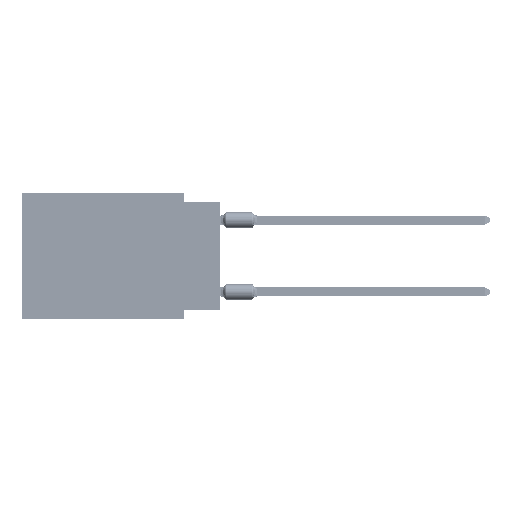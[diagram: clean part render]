
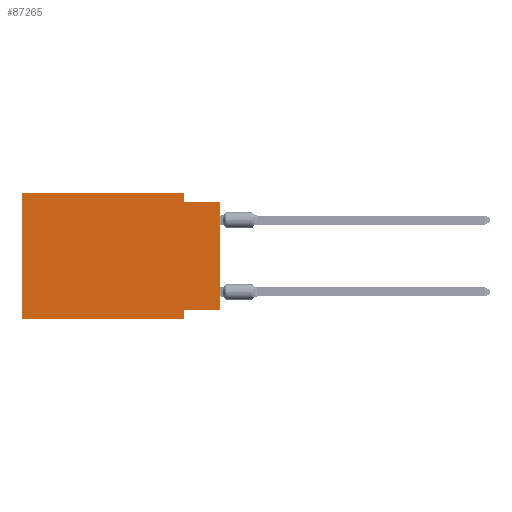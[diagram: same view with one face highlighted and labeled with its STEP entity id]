
A CAD part, left-side view. The second image highlights one B-rep face of the part: STEP entity #87265.
In plain terms, the highlighted planar face has unit normal (-1, 0, 0).
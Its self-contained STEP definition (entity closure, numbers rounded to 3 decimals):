
#952 = ORIENTED_EDGE ( 'NONE', *, *, #56576, .F. ) ;
#2219 = CARTESIAN_POINT ( 'NONE',  ( 0., 2.54, 0. ) ) ;
#2285 = LINE ( 'NONE', #32668, #85228 ) ;
#3794 = DIRECTION ( 'NONE',  ( 0., 0., -1. ) ) ;
#4928 = CARTESIAN_POINT ( 'NONE',  ( 0., 13.97, 0. ) ) ;
#5363 = VECTOR ( 'NONE', #19397, 1000. ) ;
#5784 = LINE ( 'NONE', #38015, #12832 ) ;
#7619 = EDGE_CURVE ( 'NONE', #47297, #87229, #2285, .T. ) ;
#8811 = VERTEX_POINT ( 'NONE', #83536 ) ;
#10686 = VECTOR ( 'NONE', #46884, 1000. ) ;
#11217 = DIRECTION ( 'NONE',  ( 0., 0., 1. ) ) ;
#11540 = VERTEX_POINT ( 'NONE', #43301 ) ;
#11664 = ORIENTED_EDGE ( 'NONE', *, *, #51901, .F. ) ;
#11834 = CARTESIAN_POINT ( 'NONE',  ( 0., 0., -8.255 ) ) ;
#12472 = ORIENTED_EDGE ( 'NONE', *, *, #55573, .F. ) ;
#12832 = VECTOR ( 'NONE', #90845, 1000. ) ;
#14168 = CARTESIAN_POINT ( 'NONE',  ( 0., 13.97, 0. ) ) ;
#14351 = LINE ( 'NONE', #88632, #70474 ) ;
#17151 = LINE ( 'NONE', #54526, #26824 ) ;
#19187 = CARTESIAN_POINT ( 'NONE',  ( 0., 13.97, -8.89 ) ) ;
#19397 = DIRECTION ( 'NONE',  ( 0., -1., 0. ) ) ;
#20477 = DIRECTION ( 'NONE',  ( 0., 0., -1. ) ) ;
#20645 = EDGE_CURVE ( 'NONE', #57954, #40935, #31451, .T. ) ;
#26824 = VECTOR ( 'NONE', #85425, 1000. ) ;
#27774 = EDGE_CURVE ( 'NONE', #8811, #11540, #42117, .T. ) ;
#30116 = EDGE_CURVE ( 'NONE', #36632, #11540, #65821, .T. ) ;
#31357 = ORIENTED_EDGE ( 'NONE', *, *, #20645, .F. ) ;
#31451 = LINE ( 'NONE', #38935, #10686 ) ;
#32668 = CARTESIAN_POINT ( 'NONE',  ( 0., 0., 0. ) ) ;
#36148 = DIRECTION ( 'NONE',  ( 1., 0., 0. ) ) ;
#36632 = VERTEX_POINT ( 'NONE', #53101 ) ;
#38015 = CARTESIAN_POINT ( 'NONE',  ( 0., 0., -0.635 ) ) ;
#38935 = CARTESIAN_POINT ( 'NONE',  ( 0., 2.54, 0. ) ) ;
#40935 = VERTEX_POINT ( 'NONE', #78925 ) ;
#42117 = LINE ( 'NONE', #19187, #88141 ) ;
#42158 = PLANE ( 'NONE',  #45329 ) ;
#43301 = CARTESIAN_POINT ( 'NONE',  ( 0., 2.54, -8.89 ) ) ;
#45329 = AXIS2_PLACEMENT_3D ( 'NONE', #95969, #36148, #3794 ) ;
#46884 = DIRECTION ( 'NONE',  ( 0., 0., -1. ) ) ;
#47297 = VERTEX_POINT ( 'NONE', #11834 ) ;
#51901 = EDGE_CURVE ( 'NONE', #40935, #87229, #5784, .T. ) ;
#53101 = CARTESIAN_POINT ( 'NONE',  ( 0., 2.54, -8.255 ) ) ;
#54526 = CARTESIAN_POINT ( 'NONE',  ( 0., 0., -8.255 ) ) ;
#55573 = EDGE_CURVE ( 'NONE', #8811, #68118, #14351, .T. ) ;
#56576 = EDGE_CURVE ( 'NONE', #68118, #57954, #64258, .T. ) ;
#57954 = VERTEX_POINT ( 'NONE', #2219 ) ;
#63955 = ORIENTED_EDGE ( 'NONE', *, *, #7619, .T. ) ;
#64258 = LINE ( 'NONE', #4928, #5363 ) ;
#65821 = LINE ( 'NONE', #80319, #69373 ) ;
#68118 = VERTEX_POINT ( 'NONE', #14168 ) ;
#68876 = ORIENTED_EDGE ( 'NONE', *, *, #91037, .F. ) ;
#69373 = VECTOR ( 'NONE', #20477, 1000. ) ;
#70474 = VECTOR ( 'NONE', #81152, 1000. ) ;
#72059 = FACE_OUTER_BOUND ( 'NONE', #96944, .T. ) ;
#72285 = ORIENTED_EDGE ( 'NONE', *, *, #27774, .T. ) ;
#78925 = CARTESIAN_POINT ( 'NONE',  ( 0., 2.54, -0.635 ) ) ;
#80319 = CARTESIAN_POINT ( 'NONE',  ( 0., 2.54, -8.89 ) ) ;
#81152 = DIRECTION ( 'NONE',  ( 0., 0., 1. ) ) ;
#83536 = CARTESIAN_POINT ( 'NONE',  ( 0., 13.97, -8.89 ) ) ;
#85228 = VECTOR ( 'NONE', #11217, 1000. ) ;
#85425 = DIRECTION ( 'NONE',  ( 0., 1., 0. ) ) ;
#86998 = DIRECTION ( 'NONE',  ( 0., -1., 0. ) ) ;
#87229 = VERTEX_POINT ( 'NONE', #89472 ) ;
#87265 = ADVANCED_FACE ( 'NONE', ( #72059 ), #42158, .F. ) ;
#88141 = VECTOR ( 'NONE', #86998, 1000. ) ;
#88632 = CARTESIAN_POINT ( 'NONE',  ( 0., 13.97, 0. ) ) ;
#89472 = CARTESIAN_POINT ( 'NONE',  ( 0., 0., -0.635 ) ) ;
#90845 = DIRECTION ( 'NONE',  ( 0., -1., 0. ) ) ;
#91037 = EDGE_CURVE ( 'NONE', #47297, #36632, #17151, .T. ) ;
#94386 = ORIENTED_EDGE ( 'NONE', *, *, #30116, .F. ) ;
#95969 = CARTESIAN_POINT ( 'NONE',  ( 0., 13.97, 0. ) ) ;
#96944 = EDGE_LOOP ( 'NONE', ( #63955, #11664, #31357, #952, #12472, #72285, #94386, #68876 ) ) ;
